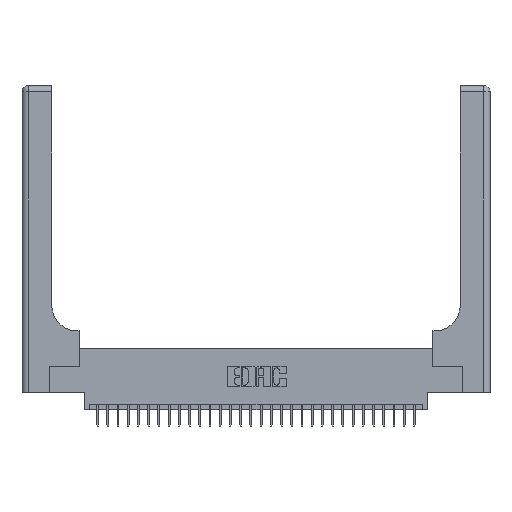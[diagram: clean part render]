
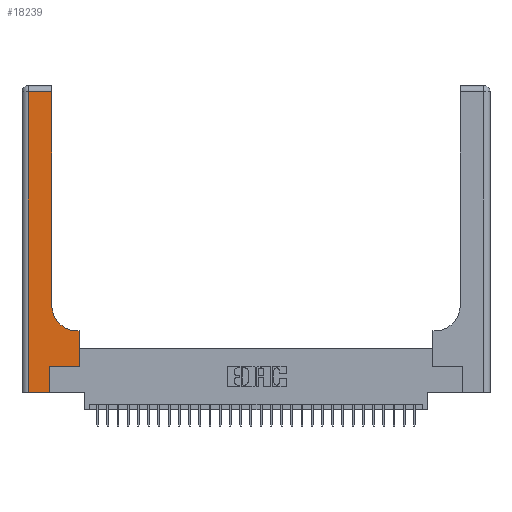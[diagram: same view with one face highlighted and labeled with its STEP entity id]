
A CAD part, top view. The second image highlights one B-rep face of the part: STEP entity #18239.
In plain terms, the highlighted planar face has unit normal (0, 0, 1).
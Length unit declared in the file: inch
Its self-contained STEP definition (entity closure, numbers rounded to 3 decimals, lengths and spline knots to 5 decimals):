
#390 = VERTEX_POINT ( 'NONE', #6700 ) ;
#805 = EDGE_CURVE ( 'NONE', #390, #20857, #16311, .T. ) ;
#1240 = CARTESIAN_POINT ( 'NONE',  ( 0.269, 0., 0.37 ) ) ;
#1337 = VERTEX_POINT ( 'NONE', #6234 ) ;
#1854 = LINE ( 'NONE', #18929, #21524 ) ;
#2302 = VERTEX_POINT ( 'NONE', #24409 ) ;
#2351 = VERTEX_POINT ( 'NONE', #22035 ) ;
#3281 = CARTESIAN_POINT ( 'NONE',  ( 0.5585, 0.6, 0.37 ) ) ;
#3520 = DIRECTION ( 'NONE',  ( 0., -1., 0. ) ) ;
#3704 = DIRECTION ( 'NONE',  ( 0., 1., 0. ) ) ;
#3886 = ORIENTED_EDGE ( 'NONE', *, *, #12638, .T. ) ;
#3954 = VECTOR ( 'NONE', #3520, 39.37008 ) ;
#4333 = CARTESIAN_POINT ( 'NONE',  ( 0.269, 0., 0.37 ) ) ;
#5021 = EDGE_CURVE ( 'NONE', #22431, #1337, #11758, .T. ) ;
#5950 = VECTOR ( 'NONE', #10935, 39.37008 ) ;
#5957 = CARTESIAN_POINT ( 'NONE',  ( 0.06, 3., 0.37 ) ) ;
#6060 = PLANE ( 'NONE',  #12555 ) ;
#6147 = ORIENTED_EDGE ( 'NONE', *, *, #16255, .T. ) ;
#6234 = CARTESIAN_POINT ( 'NONE',  ( 0.269, 0.25, 0.37 ) ) ;
#6482 = CARTESIAN_POINT ( 'NONE',  ( 0., 2.94, 0.37 ) ) ;
#6700 = CARTESIAN_POINT ( 'NONE',  ( 0.2915, 2.94, 0.37 ) ) ;
#7126 = CARTESIAN_POINT ( 'NONE',  ( 0.2915, 0.6, 0.37 ) ) ;
#7609 = CARTESIAN_POINT ( 'NONE',  ( 0.06, 2.94, 0.37 ) ) ;
#7898 = CARTESIAN_POINT ( 'NONE',  ( 0.2915, 0.85, 0.37 ) ) ;
#8296 = ORIENTED_EDGE ( 'NONE', *, *, #8720, .T. ) ;
#8720 = EDGE_CURVE ( 'NONE', #2351, #22431, #1854, .T. ) ;
#8999 = EDGE_CURVE ( 'NONE', #1337, #31037, #26112, .T. ) ;
#9083 = VECTOR ( 'NONE', #31042, 39.37008 ) ;
#9289 = CIRCLE ( 'NONE', #13691, 0.25 ) ;
#9811 = LINE ( 'NONE', #28176, #5950 ) ;
#10213 = VECTOR ( 'NONE', #12004, 39.37008 ) ;
#10935 = DIRECTION ( 'NONE',  ( 0., 1., 0. ) ) ;
#11005 = LINE ( 'NONE', #7126, #10213 ) ;
#11012 = DIRECTION ( 'NONE',  ( 0., 0., -1. ) ) ;
#11348 = CARTESIAN_POINT ( 'NONE',  ( 0.5415, 0.85, 0.37 ) ) ;
#11492 = ORIENTED_EDGE ( 'NONE', *, *, #16129, .T. ) ;
#11758 = LINE ( 'NONE', #1240, #24111 ) ;
#12004 = DIRECTION ( 'NONE',  ( -1., 0., 0. ) ) ;
#12433 = CARTESIAN_POINT ( 'NONE',  ( 0.269, 0.25, 0.37 ) ) ;
#12555 = AXIS2_PLACEMENT_3D ( 'NONE', #25782, #11012, #28257 ) ;
#12638 = EDGE_CURVE ( 'NONE', #2302, #23392, #9289, .T. ) ;
#13003 = VECTOR ( 'NONE', #17510, 39.37008 ) ;
#13691 = AXIS2_PLACEMENT_3D ( 'NONE', #11348, #28579, #13848 ) ;
#13762 = CARTESIAN_POINT ( 'NONE',  ( 0.2915, 3., 0.37 ) ) ;
#13848 = DIRECTION ( 'NONE',  ( 1., 0., 0. ) ) ;
#14070 = DIRECTION ( 'NONE',  ( 1., 0., 0. ) ) ;
#15308 = ORIENTED_EDGE ( 'NONE', *, *, #23544, .T. ) ;
#15503 = VECTOR ( 'NONE', #16450, 39.37008 ) ;
#15690 = LINE ( 'NONE', #13762, #9083 ) ;
#16129 = EDGE_CURVE ( 'NONE', #31037, #19930, #9811, .T. ) ;
#16255 = EDGE_CURVE ( 'NONE', #23392, #390, #15690, .T. ) ;
#16311 = LINE ( 'NONE', #6482, #15503 ) ;
#16450 = DIRECTION ( 'NONE',  ( -1., 0., 0. ) ) ;
#16472 = EDGE_CURVE ( 'NONE', #19930, #2302, #11005, .T. ) ;
#16810 = EDGE_LOOP ( 'NONE', ( #6147, #21464, #15308, #8296, #27985, #24294, #11492, #28346, #3886 ) ) ;
#17510 = DIRECTION ( 'NONE',  ( 1., 0., 0. ) ) ;
#18239 = ADVANCED_FACE ( 'NONE', ( #18248 ), #6060, .F. ) ;
#18248 = FACE_OUTER_BOUND ( 'NONE', #16810, .T. ) ;
#18929 = CARTESIAN_POINT ( 'NONE',  ( 0., 0., 0.37 ) ) ;
#19930 = VERTEX_POINT ( 'NONE', #3281 ) ;
#20857 = VERTEX_POINT ( 'NONE', #7609 ) ;
#21464 = ORIENTED_EDGE ( 'NONE', *, *, #805, .T. ) ;
#21524 = VECTOR ( 'NONE', #14070, 39.37008 ) ;
#22035 = CARTESIAN_POINT ( 'NONE',  ( 0.06, 0., 0.37 ) ) ;
#22431 = VERTEX_POINT ( 'NONE', #4333 ) ;
#23392 = VERTEX_POINT ( 'NONE', #7898 ) ;
#23544 = EDGE_CURVE ( 'NONE', #20857, #2351, #23606, .T. ) ;
#23606 = LINE ( 'NONE', #5957, #3954 ) ;
#24111 = VECTOR ( 'NONE', #3704, 39.37008 ) ;
#24294 = ORIENTED_EDGE ( 'NONE', *, *, #8999, .T. ) ;
#24409 = CARTESIAN_POINT ( 'NONE',  ( 0.5415, 0.6, 0.37 ) ) ;
#25782 = CARTESIAN_POINT ( 'NONE',  ( 0., 3., 0.37 ) ) ;
#26112 = LINE ( 'NONE', #12433, #13003 ) ;
#27985 = ORIENTED_EDGE ( 'NONE', *, *, #5021, .T. ) ;
#28176 = CARTESIAN_POINT ( 'NONE',  ( 0.5585, 0.25, 0.37 ) ) ;
#28257 = DIRECTION ( 'NONE',  ( -1., 0., 0. ) ) ;
#28346 = ORIENTED_EDGE ( 'NONE', *, *, #16472, .T. ) ;
#28579 = DIRECTION ( 'NONE',  ( 0., 0., -1. ) ) ;
#29199 = CARTESIAN_POINT ( 'NONE',  ( 0.5585, 0.25, 0.37 ) ) ;
#31037 = VERTEX_POINT ( 'NONE', #29199 ) ;
#31042 = DIRECTION ( 'NONE',  ( 0., 1., 0. ) ) ;
